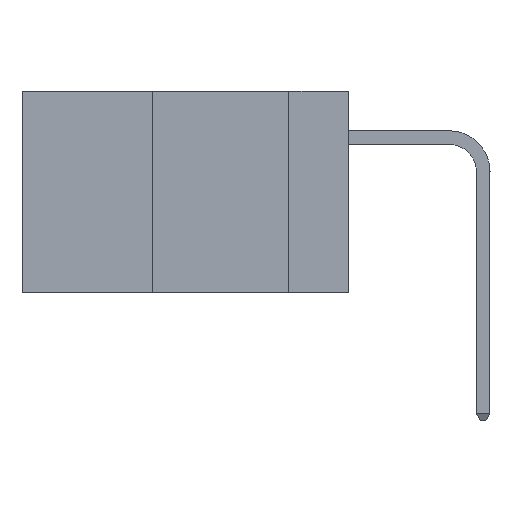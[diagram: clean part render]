
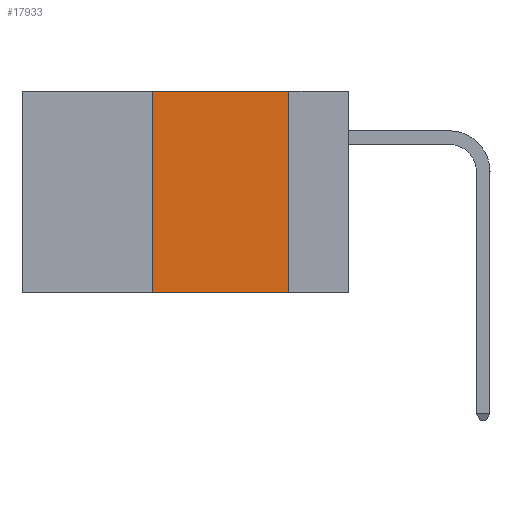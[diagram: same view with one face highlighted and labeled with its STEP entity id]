
A CAD part, left-side view. The second image highlights one B-rep face of the part: STEP entity #17933.
In plain terms, the highlighted planar face has unit normal (-1, 0, 0).
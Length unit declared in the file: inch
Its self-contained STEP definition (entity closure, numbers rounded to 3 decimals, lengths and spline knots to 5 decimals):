
#1494 = CARTESIAN_POINT ( 'NONE',  ( 0., 0.6, 0. ) ) ;
#2274 = VECTOR ( 'NONE', #4838, 39.37008 ) ;
#2605 = VECTOR ( 'NONE', #17004, 39.37008 ) ;
#3636 = VECTOR ( 'NONE', #22440, 39.37008 ) ;
#4451 = DIRECTION ( 'NONE',  ( 1., 0., 0. ) ) ;
#4838 = DIRECTION ( 'NONE',  ( 0., 0., 1. ) ) ;
#6519 = DIRECTION ( 'NONE',  ( 0., -1., 0. ) ) ;
#7865 = ORIENTED_EDGE ( 'NONE', *, *, #9855, .F. ) ;
#8375 = CARTESIAN_POINT ( 'NONE',  ( 0., 0.11, 0. ) ) ;
#9855 = EDGE_CURVE ( 'NONE', #22492, #17035, #30438, .T. ) ;
#11545 = VERTEX_POINT ( 'NONE', #17738 ) ;
#13532 = EDGE_LOOP ( 'NONE', ( #24224, #18040, #7865, #22370 ) ) ;
#14144 = CARTESIAN_POINT ( 'NONE',  ( 0., 0.6, -0.37 ) ) ;
#14773 = CARTESIAN_POINT ( 'NONE',  ( 0., 0.36, 0. ) ) ;
#17004 = DIRECTION ( 'NONE',  ( 0., -1., 0. ) ) ;
#17035 = VERTEX_POINT ( 'NONE', #14773 ) ;
#17738 = CARTESIAN_POINT ( 'NONE',  ( 0., 0.11, 0. ) ) ;
#17933 = ADVANCED_FACE ( 'NONE', ( #24931 ), #34966, .F. ) ;
#18040 = ORIENTED_EDGE ( 'NONE', *, *, #30528, .F. ) ;
#18497 = LINE ( 'NONE', #23476, #32893 ) ;
#19359 = EDGE_CURVE ( 'NONE', #22492, #32764, #32386, .T. ) ;
#21959 = CARTESIAN_POINT ( 'NONE',  ( 0., 0.36, 0. ) ) ;
#22370 = ORIENTED_EDGE ( 'NONE', *, *, #19359, .T. ) ;
#22440 = DIRECTION ( 'NONE',  ( 0., 0., -1. ) ) ;
#22492 = VERTEX_POINT ( 'NONE', #25540 ) ;
#23476 = CARTESIAN_POINT ( 'NONE',  ( 0., 0.6, 0. ) ) ;
#24224 = ORIENTED_EDGE ( 'NONE', *, *, #30266, .F. ) ;
#24272 = DIRECTION ( 'NONE',  ( 0., 0., -1. ) ) ;
#24931 = FACE_OUTER_BOUND ( 'NONE', #13532, .T. ) ;
#25341 = LINE ( 'NONE', #8375, #3636 ) ;
#25540 = CARTESIAN_POINT ( 'NONE',  ( 0., 0.36, -0.37 ) ) ;
#30266 = EDGE_CURVE ( 'NONE', #11545, #32764, #25341, .T. ) ;
#30438 = LINE ( 'NONE', #21959, #2274 ) ;
#30528 = EDGE_CURVE ( 'NONE', #17035, #11545, #18497, .T. ) ;
#32386 = LINE ( 'NONE', #14144, #2605 ) ;
#32764 = VERTEX_POINT ( 'NONE', #33693 ) ;
#32893 = VECTOR ( 'NONE', #6519, 39.37008 ) ;
#33693 = CARTESIAN_POINT ( 'NONE',  ( 0., 0.11, -0.37 ) ) ;
#34966 = PLANE ( 'NONE',  #36099 ) ;
#36099 = AXIS2_PLACEMENT_3D ( 'NONE', #1494, #4451, #24272 ) ;
